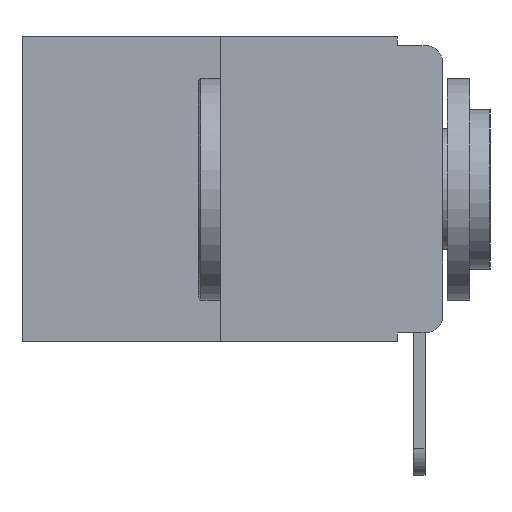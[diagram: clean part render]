
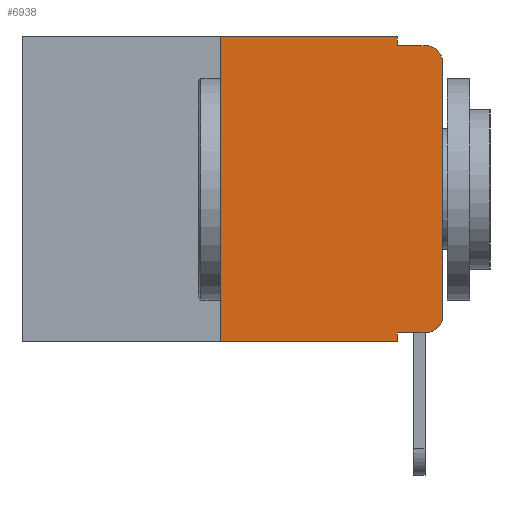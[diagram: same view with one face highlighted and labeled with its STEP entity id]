
A CAD part, left-side view. The second image highlights one B-rep face of the part: STEP entity #6938.
In plain terms, the highlighted planar face has unit normal (-1, 0, 0).
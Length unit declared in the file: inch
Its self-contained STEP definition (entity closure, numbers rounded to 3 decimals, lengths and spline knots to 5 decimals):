
#76 = CARTESIAN_POINT ( 'NONE',  ( 0., 0.25, 0. ) ) ;
#149 = AXIS2_PLACEMENT_3D ( 'NONE', #7592, #21580, #9633 ) ;
#207 = LINE ( 'NONE', #14584, #859 ) ;
#644 = AXIS2_PLACEMENT_3D ( 'NONE', #25467, #5522, #19619 ) ;
#668 = VERTEX_POINT ( 'NONE', #11695 ) ;
#814 = LINE ( 'NONE', #4340, #16640 ) ;
#834 = VECTOR ( 'NONE', #20557, 39.37008 ) ;
#859 = VECTOR ( 'NONE', #16564, 39.37008 ) ;
#1231 = VERTEX_POINT ( 'NONE', #19773 ) ;
#1816 = DIRECTION ( 'NONE',  ( 0., -1., 0. ) ) ;
#2186 = VERTEX_POINT ( 'NONE', #3669 ) ;
#2961 = EDGE_CURVE ( 'NONE', #1231, #14637, #3282, .T. ) ;
#2995 = CARTESIAN_POINT ( 'NONE',  ( 0., 0.051, 0. ) ) ;
#3185 = ORIENTED_EDGE ( 'NONE', *, *, #9184, .T. ) ;
#3266 = LINE ( 'NONE', #16204, #17591 ) ;
#3282 = LINE ( 'NONE', #23050, #14854 ) ;
#3424 = PLANE ( 'NONE',  #644 ) ;
#3619 = VECTOR ( 'NONE', #9018, 39.37008 ) ;
#3669 = CARTESIAN_POINT ( 'NONE',  ( 0., 0., -0.03 ) ) ;
#4340 = CARTESIAN_POINT ( 'NONE',  ( 0., 0.473, 0. ) ) ;
#4649 = CIRCLE ( 'NONE', #6142, 0.02 ) ;
#4704 = VERTEX_POINT ( 'NONE', #12135 ) ;
#5522 = DIRECTION ( 'NONE',  ( 1., 0., 0. ) ) ;
#5662 = VECTOR ( 'NONE', #24023, 39.37008 ) ;
#6142 = AXIS2_PLACEMENT_3D ( 'NONE', #20260, #8271, #22234 ) ;
#6518 = LINE ( 'NONE', #76, #834 ) ;
#6577 = ORIENTED_EDGE ( 'NONE', *, *, #24529, .T. ) ;
#6644 = EDGE_CURVE ( 'NONE', #20601, #4704, #207, .T. ) ;
#6938 = ADVANCED_FACE ( 'NONE', ( #18506 ), #3424, .F. ) ;
#7592 = CARTESIAN_POINT ( 'NONE',  ( 0., 0.02, -0.313 ) ) ;
#8131 = ORIENTED_EDGE ( 'NONE', *, *, #11947, .T. ) ;
#8271 = DIRECTION ( 'NONE',  ( -1., 0., 0. ) ) ;
#8347 = EDGE_LOOP ( 'NONE', ( #6577, #8131, #8777, #9651, #10202, #10422, #14638, #14030, #10125, #3185 ) ) ;
#8777 = ORIENTED_EDGE ( 'NONE', *, *, #20100, .F. ) ;
#9018 = DIRECTION ( 'NONE',  ( 0., 0., 1. ) ) ;
#9184 = EDGE_CURVE ( 'NONE', #17958, #14052, #16247, .T. ) ;
#9253 = CARTESIAN_POINT ( 'NONE',  ( 0., 0.051, -0.01 ) ) ;
#9633 = DIRECTION ( 'NONE',  ( 0., 0., -1. ) ) ;
#9651 = ORIENTED_EDGE ( 'NONE', *, *, #6644, .F. ) ;
#10125 = ORIENTED_EDGE ( 'NONE', *, *, #22029, .T. ) ;
#10202 = ORIENTED_EDGE ( 'NONE', *, *, #13074, .F. ) ;
#10422 = ORIENTED_EDGE ( 'NONE', *, *, #24401, .F. ) ;
#10617 = VECTOR ( 'NONE', #25169, 39.37008 ) ;
#11695 = CARTESIAN_POINT ( 'NONE',  ( 0., 0.02, -0.01 ) ) ;
#11947 = EDGE_CURVE ( 'NONE', #2186, #668, #4649, .T. ) ;
#12135 = CARTESIAN_POINT ( 'NONE',  ( 0., 0.051, -0.01 ) ) ;
#13074 = EDGE_CURVE ( 'NONE', #19143, #20601, #814, .T. ) ;
#14030 = ORIENTED_EDGE ( 'NONE', *, *, #2961, .F. ) ;
#14052 = VERTEX_POINT ( 'NONE', #18131 ) ;
#14228 = CARTESIAN_POINT ( 'NONE',  ( 0., 0.051, -0.333 ) ) ;
#14584 = CARTESIAN_POINT ( 'NONE',  ( 0., 0.051, 0. ) ) ;
#14637 = VERTEX_POINT ( 'NONE', #21695 ) ;
#14638 = ORIENTED_EDGE ( 'NONE', *, *, #18906, .T. ) ;
#14767 = CARTESIAN_POINT ( 'NONE',  ( 0., 0.25, -0.343 ) ) ;
#14854 = VECTOR ( 'NONE', #15766, 39.37008 ) ;
#15766 = DIRECTION ( 'NONE',  ( 0., 0., -1. ) ) ;
#16204 = CARTESIAN_POINT ( 'NONE',  ( 0., 0.473, -0.343 ) ) ;
#16247 = CIRCLE ( 'NONE', #149, 0.02 ) ;
#16564 = DIRECTION ( 'NONE',  ( 0., 0., -1. ) ) ;
#16640 = VECTOR ( 'NONE', #26251, 39.37008 ) ;
#17102 = CARTESIAN_POINT ( 'NONE',  ( 0., 0.02, -0.333 ) ) ;
#17591 = VECTOR ( 'NONE', #1816, 39.37008 ) ;
#17958 = VERTEX_POINT ( 'NONE', #17102 ) ;
#18131 = CARTESIAN_POINT ( 'NONE',  ( 0., 0., -0.313 ) ) ;
#18506 = FACE_OUTER_BOUND ( 'NONE', #8347, .T. ) ;
#18906 = EDGE_CURVE ( 'NONE', #25477, #14637, #3266, .T. ) ;
#19143 = VERTEX_POINT ( 'NONE', #22899 ) ;
#19619 = DIRECTION ( 'NONE',  ( 0., 0., -1. ) ) ;
#19773 = CARTESIAN_POINT ( 'NONE',  ( 0., 0.051, -0.333 ) ) ;
#20100 = EDGE_CURVE ( 'NONE', #4704, #668, #21197, .T. ) ;
#20260 = CARTESIAN_POINT ( 'NONE',  ( 0., 0.02, -0.03 ) ) ;
#20557 = DIRECTION ( 'NONE',  ( 0., 0., 1. ) ) ;
#20601 = VERTEX_POINT ( 'NONE', #2995 ) ;
#20993 = CARTESIAN_POINT ( 'NONE',  ( 0., 0., 0. ) ) ;
#21197 = LINE ( 'NONE', #9253, #10617 ) ;
#21580 = DIRECTION ( 'NONE',  ( -1., 0., 0. ) ) ;
#21684 = LINE ( 'NONE', #14228, #5662 ) ;
#21695 = CARTESIAN_POINT ( 'NONE',  ( 0., 0.051, -0.343 ) ) ;
#22029 = EDGE_CURVE ( 'NONE', #1231, #17958, #21684, .T. ) ;
#22234 = DIRECTION ( 'NONE',  ( 0., 0., -1. ) ) ;
#22899 = CARTESIAN_POINT ( 'NONE',  ( 0., 0.25, 0. ) ) ;
#23050 = CARTESIAN_POINT ( 'NONE',  ( 0., 0.051, 0. ) ) ;
#24023 = DIRECTION ( 'NONE',  ( 0., -1., 0. ) ) ;
#24401 = EDGE_CURVE ( 'NONE', #25477, #19143, #6518, .T. ) ;
#24529 = EDGE_CURVE ( 'NONE', #14052, #2186, #24999, .T. ) ;
#24999 = LINE ( 'NONE', #20993, #3619 ) ;
#25169 = DIRECTION ( 'NONE',  ( 0., -1., 0. ) ) ;
#25467 = CARTESIAN_POINT ( 'NONE',  ( 0., 0.473, 0. ) ) ;
#25477 = VERTEX_POINT ( 'NONE', #14767 ) ;
#26251 = DIRECTION ( 'NONE',  ( 0., -1., 0. ) ) ;
